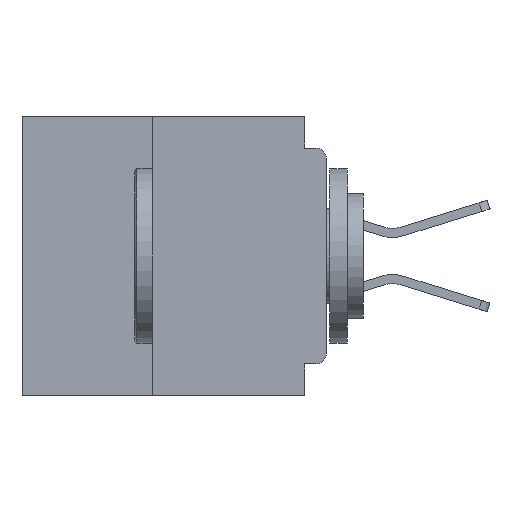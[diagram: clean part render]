
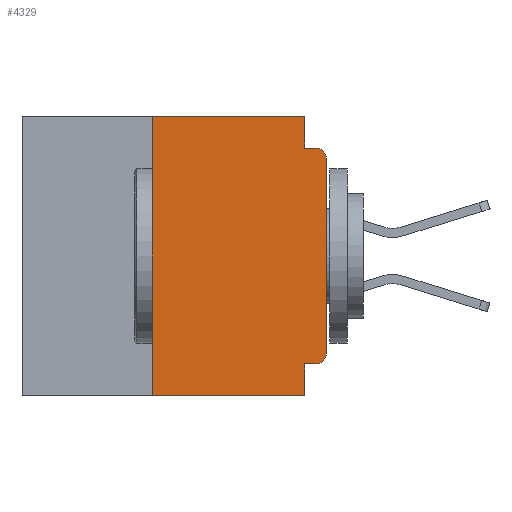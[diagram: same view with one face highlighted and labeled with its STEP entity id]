
A CAD part, left-side view. The second image highlights one B-rep face of the part: STEP entity #4329.
In plain terms, the highlighted planar face has unit normal (-1, 0, 0).
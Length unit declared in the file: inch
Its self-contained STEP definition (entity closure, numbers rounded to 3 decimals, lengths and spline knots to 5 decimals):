
#291 = ORIENTED_EDGE ( 'NONE', *, *, #21247, .F. ) ;
#677 = CARTESIAN_POINT ( 'NONE',  ( 0., 0.031, -0.355 ) ) ;
#1615 = DIRECTION ( 'NONE',  ( -1., 0., 0. ) ) ;
#1724 = CARTESIAN_POINT ( 'NONE',  ( 0., 0.031, -0.045 ) ) ;
#2219 = VERTEX_POINT ( 'NONE', #9078 ) ;
#2450 = VERTEX_POINT ( 'NONE', #23174 ) ;
#3240 = EDGE_LOOP ( 'NONE', ( #22836, #31552, #22847, #36528, #291, #18110, #19194, #35096, #34222, #24792 ) ) ;
#4276 = LINE ( 'NONE', #36019, #21429 ) ;
#4329 = ADVANCED_FACE ( 'NONE', ( #38122 ), #16502, .F. ) ;
#4357 = LINE ( 'NONE', #7758, #27658 ) ;
#4553 = CIRCLE ( 'NONE', #36079, 0.015 ) ;
#4998 = EDGE_CURVE ( 'NONE', #37934, #15513, #4553, .T. ) ;
#5810 = DIRECTION ( 'NONE',  ( 0., -1., 0. ) ) ;
#7344 = LINE ( 'NONE', #38785, #14419 ) ;
#7758 = CARTESIAN_POINT ( 'NONE',  ( 0., 0.031, -0.4 ) ) ;
#8166 = AXIS2_PLACEMENT_3D ( 'NONE', #19936, #1615, #23035 ) ;
#8573 = VECTOR ( 'NONE', #5810, 39.37008 ) ;
#9078 = CARTESIAN_POINT ( 'NONE',  ( 0., 0.25, -0.4 ) ) ;
#9467 = EDGE_CURVE ( 'NONE', #16160, #15513, #17547, .T. ) ;
#9485 = CARTESIAN_POINT ( 'NONE',  ( 0., 0.031, 0. ) ) ;
#10653 = DIRECTION ( 'NONE',  ( 0., -1., 0. ) ) ;
#11772 = LINE ( 'NONE', #15278, #34781 ) ;
#11938 = CARTESIAN_POINT ( 'NONE',  ( 0., 0., -0.045 ) ) ;
#12513 = DIRECTION ( 'NONE',  ( 0., 0., -1. ) ) ;
#12704 = CARTESIAN_POINT ( 'NONE',  ( 0., 0.25, 0. ) ) ;
#13471 = AXIS2_PLACEMENT_3D ( 'NONE', #17263, #16462, #16454 ) ;
#13788 = VERTEX_POINT ( 'NONE', #12704 ) ;
#14419 = VECTOR ( 'NONE', #24072, 39.37008 ) ;
#14698 = LINE ( 'NONE', #9485, #29872 ) ;
#14824 = EDGE_CURVE ( 'NONE', #2219, #13788, #7344, .T. ) ;
#15278 = CARTESIAN_POINT ( 'NONE',  ( 0., 0.437, 0. ) ) ;
#15513 = VERTEX_POINT ( 'NONE', #17002 ) ;
#15612 = VECTOR ( 'NONE', #10653, 39.37008 ) ;
#16160 = VERTEX_POINT ( 'NONE', #1724 ) ;
#16454 = DIRECTION ( 'NONE',  ( 0., 0., -1. ) ) ;
#16462 = DIRECTION ( 'NONE',  ( 1., 0., 0. ) ) ;
#16502 = PLANE ( 'NONE',  #13471 ) ;
#17002 = CARTESIAN_POINT ( 'NONE',  ( 0., 0.015, -0.045 ) ) ;
#17263 = CARTESIAN_POINT ( 'NONE',  ( 0., 0.437, 0. ) ) ;
#17547 = LINE ( 'NONE', #11938, #8573 ) ;
#17865 = VECTOR ( 'NONE', #34476, 39.37008 ) ;
#17965 = CARTESIAN_POINT ( 'NONE',  ( 0., 0.031, 0. ) ) ;
#18060 = CIRCLE ( 'NONE', #8166, 0.015 ) ;
#18104 = DIRECTION ( 'NONE',  ( 0., 1., 0. ) ) ;
#18110 = ORIENTED_EDGE ( 'NONE', *, *, #14824, .F. ) ;
#18325 = VERTEX_POINT ( 'NONE', #34678 ) ;
#18336 = EDGE_CURVE ( 'NONE', #2450, #31169, #18060, .T. ) ;
#19194 = ORIENTED_EDGE ( 'NONE', *, *, #20246, .T. ) ;
#19936 = CARTESIAN_POINT ( 'NONE',  ( 0., 0.015, -0.34 ) ) ;
#20246 = EDGE_CURVE ( 'NONE', #2219, #18325, #31671, .T. ) ;
#21247 = EDGE_CURVE ( 'NONE', #13788, #25668, #11772, .T. ) ;
#21429 = VECTOR ( 'NONE', #18104, 39.37008 ) ;
#22836 = ORIENTED_EDGE ( 'NONE', *, *, #25995, .T. ) ;
#22847 = ORIENTED_EDGE ( 'NONE', *, *, #9467, .F. ) ;
#23035 = DIRECTION ( 'NONE',  ( 0., 0., -1. ) ) ;
#23174 = CARTESIAN_POINT ( 'NONE',  ( 0., 0.015, -0.355 ) ) ;
#23436 = DIRECTION ( 'NONE',  ( 0., 0., -1. ) ) ;
#23511 = DIRECTION ( 'NONE',  ( -1., 0., 0. ) ) ;
#23651 = CARTESIAN_POINT ( 'NONE',  ( 0., 0.015, -0.06 ) ) ;
#24072 = DIRECTION ( 'NONE',  ( 0., 0., 1. ) ) ;
#24498 = EDGE_CURVE ( 'NONE', #25668, #16160, #14698, .T. ) ;
#24787 = CARTESIAN_POINT ( 'NONE',  ( 0., 0., -0.06 ) ) ;
#24792 = ORIENTED_EDGE ( 'NONE', *, *, #18336, .T. ) ;
#25668 = VERTEX_POINT ( 'NONE', #17965 ) ;
#25953 = DIRECTION ( 'NONE',  ( 0., 0., -1. ) ) ;
#25995 = EDGE_CURVE ( 'NONE', #31169, #37934, #26035, .T. ) ;
#26035 = LINE ( 'NONE', #31539, #17865 ) ;
#27510 = CARTESIAN_POINT ( 'NONE',  ( 0., 0., -0.34 ) ) ;
#27658 = VECTOR ( 'NONE', #25953, 39.37008 ) ;
#28337 = VERTEX_POINT ( 'NONE', #677 ) ;
#28802 = CARTESIAN_POINT ( 'NONE',  ( 0., 0.437, -0.4 ) ) ;
#29872 = VECTOR ( 'NONE', #12513, 39.37008 ) ;
#30487 = DIRECTION ( 'NONE',  ( 0., -1., 0. ) ) ;
#31169 = VERTEX_POINT ( 'NONE', #27510 ) ;
#31539 = CARTESIAN_POINT ( 'NONE',  ( 0., 0., 0. ) ) ;
#31552 = ORIENTED_EDGE ( 'NONE', *, *, #4998, .T. ) ;
#31671 = LINE ( 'NONE', #28802, #15612 ) ;
#34222 = ORIENTED_EDGE ( 'NONE', *, *, #37175, .F. ) ;
#34476 = DIRECTION ( 'NONE',  ( 0., 0., 1. ) ) ;
#34678 = CARTESIAN_POINT ( 'NONE',  ( 0., 0.031, -0.4 ) ) ;
#34781 = VECTOR ( 'NONE', #30487, 39.37008 ) ;
#35096 = ORIENTED_EDGE ( 'NONE', *, *, #36267, .F. ) ;
#36019 = CARTESIAN_POINT ( 'NONE',  ( 0., 0., -0.355 ) ) ;
#36079 = AXIS2_PLACEMENT_3D ( 'NONE', #23651, #23511, #23436 ) ;
#36267 = EDGE_CURVE ( 'NONE', #28337, #18325, #4357, .T. ) ;
#36528 = ORIENTED_EDGE ( 'NONE', *, *, #24498, .F. ) ;
#37175 = EDGE_CURVE ( 'NONE', #2450, #28337, #4276, .T. ) ;
#37934 = VERTEX_POINT ( 'NONE', #24787 ) ;
#38122 = FACE_OUTER_BOUND ( 'NONE', #3240, .T. ) ;
#38785 = CARTESIAN_POINT ( 'NONE',  ( 0., 0.25, -0.4 ) ) ;
